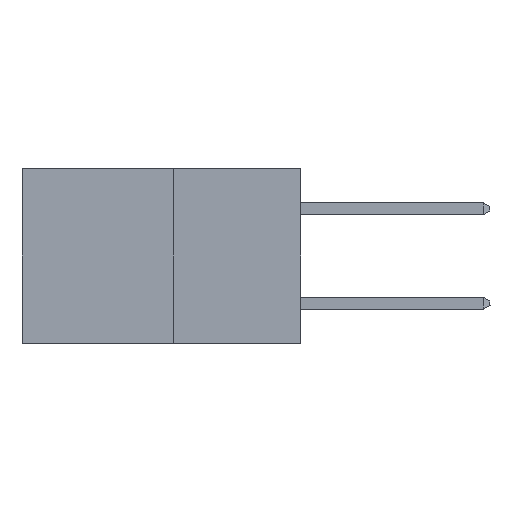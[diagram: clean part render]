
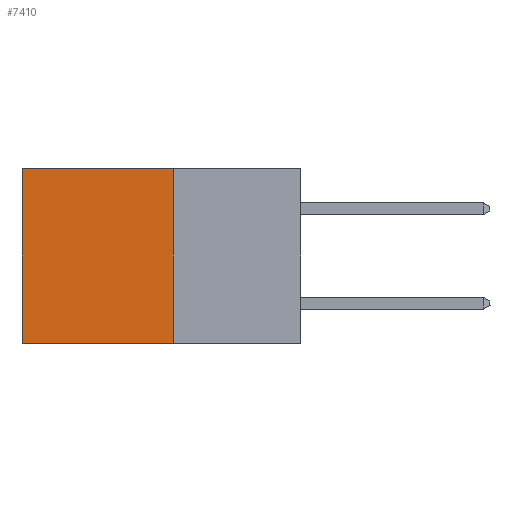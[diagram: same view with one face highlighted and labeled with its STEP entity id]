
A CAD part, left-side view. The second image highlights one B-rep face of the part: STEP entity #7410.
In plain terms, the highlighted planar face has unit normal (-1, 0, 0).
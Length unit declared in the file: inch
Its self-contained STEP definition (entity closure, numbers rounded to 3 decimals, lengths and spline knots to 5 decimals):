
#195 = CARTESIAN_POINT ( 'NONE',  ( 0.277, 0.59, 0. ) ) ;
#219 = CARTESIAN_POINT ( 'NONE',  ( 0.277, 0.27, 0. ) ) ;
#1136 = EDGE_CURVE ( 'NONE', #7480, #5688, #2729, .T. ) ;
#1151 = DIRECTION ( 'NONE',  ( 0., 1., 0. ) ) ;
#1158 = DIRECTION ( 'NONE',  ( 0., 0., -1. ) ) ;
#1177 = EDGE_CURVE ( 'NONE', #7480, #15534, #12772, .T. ) ;
#1819 = FACE_OUTER_BOUND ( 'NONE', #15749, .T. ) ;
#2465 = CARTESIAN_POINT ( 'NONE',  ( 0.277, 0.27, -0.37 ) ) ;
#2729 = LINE ( 'NONE', #7201, #3126 ) ;
#2846 = ORIENTED_EDGE ( 'NONE', *, *, #3154, .T. ) ;
#3002 = VERTEX_POINT ( 'NONE', #14029 ) ;
#3126 = VECTOR ( 'NONE', #11773, 39.37008 ) ;
#3154 = EDGE_CURVE ( 'NONE', #15534, #3002, #7011, .T. ) ;
#3896 = CARTESIAN_POINT ( 'NONE',  ( 0.277, 0.27, -0.37 ) ) ;
#3910 = VECTOR ( 'NONE', #1151, 39.37008 ) ;
#4154 = DIRECTION ( 'NONE',  ( 0., 1., 0. ) ) ;
#4324 = LINE ( 'NONE', #3896, #3910 ) ;
#4820 = ORIENTED_EDGE ( 'NONE', *, *, #1136, .F. ) ;
#5304 = VECTOR ( 'NONE', #4154, 39.37008 ) ;
#5688 = VERTEX_POINT ( 'NONE', #2465 ) ;
#6193 = CARTESIAN_POINT ( 'NONE',  ( 0.277, 0.27, -0.37 ) ) ;
#6356 = CARTESIAN_POINT ( 'NONE',  ( 0.277, 0.27, 0. ) ) ;
#7011 = LINE ( 'NONE', #8040, #13299 ) ;
#7201 = CARTESIAN_POINT ( 'NONE',  ( 0.277, 0.27, -0.37 ) ) ;
#7410 = ADVANCED_FACE ( 'NONE', ( #1819 ), #16224, .F. ) ;
#7480 = VERTEX_POINT ( 'NONE', #6356 ) ;
#8040 = CARTESIAN_POINT ( 'NONE',  ( 0.277, 0.59, -0.37 ) ) ;
#8099 = AXIS2_PLACEMENT_3D ( 'NONE', #6193, #8712, #1158 ) ;
#8213 = ORIENTED_EDGE ( 'NONE', *, *, #9691, .F. ) ;
#8712 = DIRECTION ( 'NONE',  ( 1., 0., 0. ) ) ;
#9306 = DIRECTION ( 'NONE',  ( 0., 0., -1. ) ) ;
#9691 = EDGE_CURVE ( 'NONE', #5688, #3002, #4324, .T. ) ;
#11773 = DIRECTION ( 'NONE',  ( 0., 0., -1. ) ) ;
#12772 = LINE ( 'NONE', #219, #5304 ) ;
#12914 = ORIENTED_EDGE ( 'NONE', *, *, #1177, .T. ) ;
#13299 = VECTOR ( 'NONE', #9306, 39.37008 ) ;
#14029 = CARTESIAN_POINT ( 'NONE',  ( 0.277, 0.59, -0.37 ) ) ;
#15534 = VERTEX_POINT ( 'NONE', #195 ) ;
#15749 = EDGE_LOOP ( 'NONE', ( #2846, #8213, #4820, #12914 ) ) ;
#16224 = PLANE ( 'NONE',  #8099 ) ;
